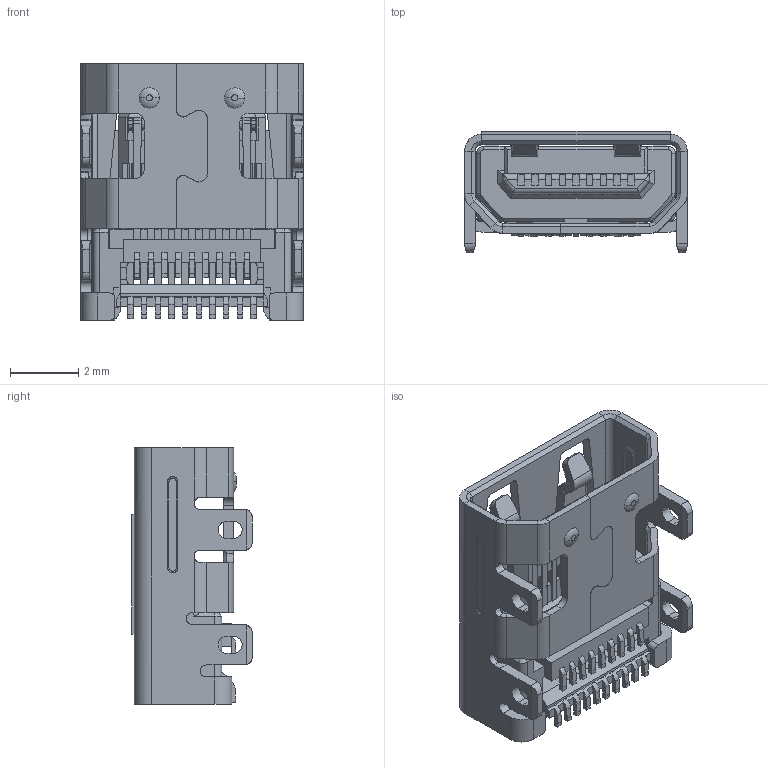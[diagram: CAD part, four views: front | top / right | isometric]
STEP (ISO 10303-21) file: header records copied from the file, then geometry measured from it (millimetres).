
FILE_DESCRIPTION (( 'STEP AP214' ), '1' );
FILE_NAME ('694H319-162-211.STEP', '2021-01-13T18:40:54', ( '' ), ( '' ), 'SwSTEP 2.0', 'SolidWorks 2020', '' );
FILE_SCHEMA (( 'AUTOMOTIVE_DESIGN' ));
Length unit declared in the file: millimetre
Products named in the file (4): Tape 694H319-X62-211; Insulator 694H319-X62-211; Shell 694H319-X62-211; 694H319-162-211
Assembly tree (3 placements, depth 2):
  694H319-162-211
    Insulator 694H319-X62-211
    Shell 694H319-X62-211
    Tape 694H319-X62-211
Bounding box: 6.5 x 3.53 x 7.5 mm (x, y, z)
Volume: 61.9 mm3; surface area: 457 mm2
Topology: 3 solids, 3 shells, 1440 faces, 4194 edges, 2681 vertices
Faces by surface type: plane 1147, cylinder 218, cone 40, bspline 35
Entity records: 61871 total; most frequent: CARTESIAN_POINT 14117, ORIENTED_EDGE 8386, DIRECTION 6306, EDGE_CURVE 4193, VECTOR 3182, LINE 3182, VERTEX_POINT 2681, AXIS2_PLACEMENT_3D 1562
